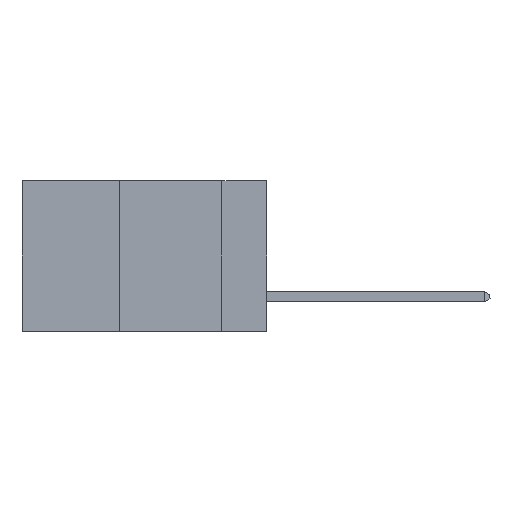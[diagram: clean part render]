
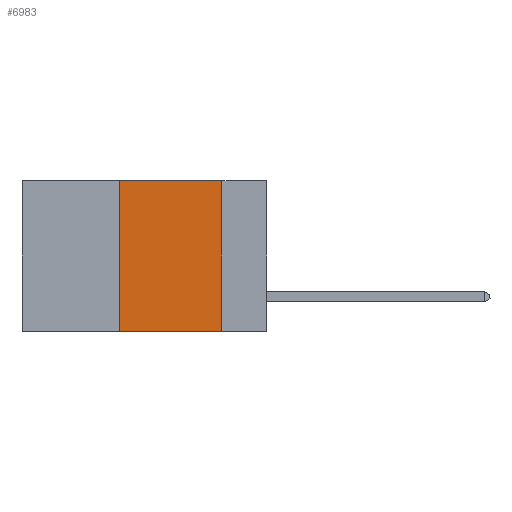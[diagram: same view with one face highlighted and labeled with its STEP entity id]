
A CAD part, left-side view. The second image highlights one B-rep face of the part: STEP entity #6983.
In plain terms, the highlighted planar face has unit normal (-1, 0, 0).
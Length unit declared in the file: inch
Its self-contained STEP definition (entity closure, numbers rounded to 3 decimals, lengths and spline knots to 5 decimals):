
#129 = CARTESIAN_POINT ( 'NONE',  ( 0., 0.6, 0. ) ) ;
#528 = CARTESIAN_POINT ( 'NONE',  ( 0., 0.11, 0. ) ) ;
#1427 = VECTOR ( 'NONE', #10789, 39.37008 ) ;
#1547 = ORIENTED_EDGE ( 'NONE', *, *, #2282, .F. ) ;
#1611 = CARTESIAN_POINT ( 'NONE',  ( 0., 0.11, 0. ) ) ;
#1811 = VERTEX_POINT ( 'NONE', #1611 ) ;
#1857 = DIRECTION ( 'NONE',  ( 0., 0., -1. ) ) ;
#1924 = VERTEX_POINT ( 'NONE', #9210 ) ;
#2023 = EDGE_CURVE ( 'NONE', #12004, #1924, #11722, .T. ) ;
#2282 = EDGE_CURVE ( 'NONE', #1811, #4570, #5569, .T. ) ;
#2346 = ORIENTED_EDGE ( 'NONE', *, *, #10753, .T. ) ;
#2719 = DIRECTION ( 'NONE',  ( 0., 0., -1. ) ) ;
#3987 = CARTESIAN_POINT ( 'NONE',  ( 0., 0.36, -0.37 ) ) ;
#4176 = CARTESIAN_POINT ( 'NONE',  ( 0., 0.6, -0.37 ) ) ;
#4476 = CARTESIAN_POINT ( 'NONE',  ( 0., 0.36, 0. ) ) ;
#4570 = VERTEX_POINT ( 'NONE', #5526 ) ;
#4702 = ORIENTED_EDGE ( 'NONE', *, *, #2023, .F. ) ;
#5094 = VECTOR ( 'NONE', #5220, 39.37008 ) ;
#5220 = DIRECTION ( 'NONE',  ( 0., -1., 0. ) ) ;
#5351 = EDGE_LOOP ( 'NONE', ( #1547, #12575, #4702, #2346 ) ) ;
#5526 = CARTESIAN_POINT ( 'NONE',  ( 0., 0.11, -0.37 ) ) ;
#5569 = LINE ( 'NONE', #528, #7432 ) ;
#6087 = VECTOR ( 'NONE', #9805, 39.37008 ) ;
#6983 = ADVANCED_FACE ( 'NONE', ( #12527 ), #10320, .F. ) ;
#7113 = LINE ( 'NONE', #129, #1427 ) ;
#7182 = CARTESIAN_POINT ( 'NONE',  ( 0., 0.6, 0. ) ) ;
#7432 = VECTOR ( 'NONE', #2719, 39.37008 ) ;
#8235 = DIRECTION ( 'NONE',  ( 1., 0., 0. ) ) ;
#8271 = LINE ( 'NONE', #4176, #5094 ) ;
#9210 = CARTESIAN_POINT ( 'NONE',  ( 0., 0.36, 0. ) ) ;
#9805 = DIRECTION ( 'NONE',  ( 0., 0., 1. ) ) ;
#10320 = PLANE ( 'NONE',  #12444 ) ;
#10753 = EDGE_CURVE ( 'NONE', #12004, #4570, #8271, .T. ) ;
#10789 = DIRECTION ( 'NONE',  ( 0., -1., 0. ) ) ;
#11722 = LINE ( 'NONE', #4476, #6087 ) ;
#12004 = VERTEX_POINT ( 'NONE', #3987 ) ;
#12353 = EDGE_CURVE ( 'NONE', #1924, #1811, #7113, .T. ) ;
#12444 = AXIS2_PLACEMENT_3D ( 'NONE', #7182, #8235, #1857 ) ;
#12527 = FACE_OUTER_BOUND ( 'NONE', #5351, .T. ) ;
#12575 = ORIENTED_EDGE ( 'NONE', *, *, #12353, .F. ) ;
